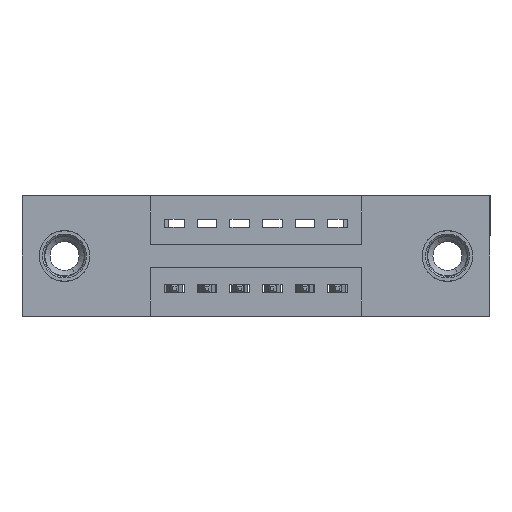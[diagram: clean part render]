
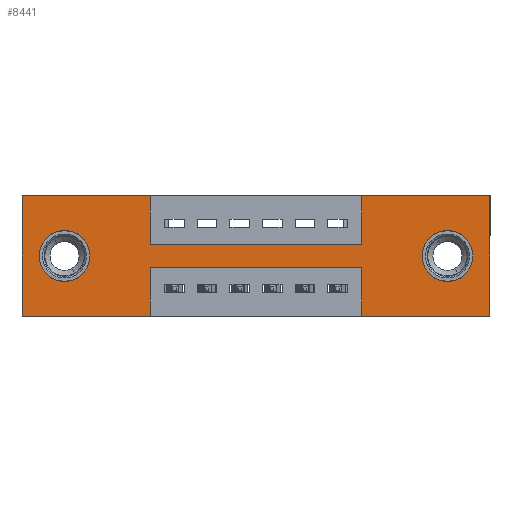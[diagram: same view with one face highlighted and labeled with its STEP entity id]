
A CAD part, front view. The second image highlights one B-rep face of the part: STEP entity #8441.
In plain terms, the highlighted planar face has unit normal (0, -1, 0).
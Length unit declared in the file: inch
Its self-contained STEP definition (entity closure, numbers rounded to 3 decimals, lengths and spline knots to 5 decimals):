
#17 = DIRECTION ( 'NONE',  ( 0., 0., 1. ) ) ;
#124 = DIRECTION ( 'NONE',  ( -1., 0., 0. ) ) ;
#183 = DIRECTION ( 'NONE',  ( -1., 0., 0. ) ) ;
#282 = EDGE_CURVE ( 'NONE', #2676, #2410, #8455, .T. ) ;
#309 = VERTEX_POINT ( 'NONE', #11609 ) ;
#420 = EDGE_CURVE ( 'NONE', #2410, #4218, #13909, .T. ) ;
#437 = EDGE_CURVE ( 'NONE', #10098, #4609, #4010, .T. ) ;
#442 = VERTEX_POINT ( 'NONE', #10493 ) ;
#476 = FACE_BOUND ( 'NONE', #6286, .T. ) ;
#587 = AXIS2_PLACEMENT_3D ( 'NONE', #9473, #10559, #1787 ) ;
#593 = LINE ( 'NONE', #3396, #13735 ) ;
#635 = FACE_OUTER_BOUND ( 'NONE', #5499, .T. ) ;
#681 = EDGE_CURVE ( 'NONE', #6985, #309, #10840, .T. ) ;
#711 = DIRECTION ( 'NONE',  ( 1., 0., 0. ) ) ;
#833 = FACE_BOUND ( 'NONE', #12904, .T. ) ;
#1046 = CARTESIAN_POINT ( 'NONE',  ( 1.0425, 0., 0. ) ) ;
#1182 = CARTESIAN_POINT ( 'NONE',  ( 0., 0., -0.37 ) ) ;
#1187 = DIRECTION ( 'NONE',  ( 0., 0., 1. ) ) ;
#1253 = EDGE_CURVE ( 'NONE', #4609, #10098, #2967, .T. ) ;
#1404 = CARTESIAN_POINT ( 'NONE',  ( 0.3925, 0., -0.15 ) ) ;
#1427 = EDGE_CURVE ( 'NONE', #4858, #3774, #3462, .T. ) ;
#1657 = VECTOR ( 'NONE', #2390, 39.37008 ) ;
#1787 = DIRECTION ( 'NONE',  ( 0., 0., -1. ) ) ;
#1828 = ORIENTED_EDGE ( 'NONE', *, *, #282, .F. ) ;
#1973 = VECTOR ( 'NONE', #4788, 39.37008 ) ;
#1985 = EDGE_CURVE ( 'NONE', #11065, #4858, #8744, .T. ) ;
#2332 = VECTOR ( 'NONE', #13837, 39.37008 ) ;
#2390 = DIRECTION ( 'NONE',  ( 1., 0., 0. ) ) ;
#2410 = VERTEX_POINT ( 'NONE', #1046 ) ;
#2585 = LINE ( 'NONE', #5685, #11122 ) ;
#2676 = VERTEX_POINT ( 'NONE', #9174 ) ;
#2867 = CARTESIAN_POINT ( 'NONE',  ( 0., 0., 0. ) ) ;
#2967 = CIRCLE ( 'NONE', #7599, 0.078 ) ;
#3246 = CARTESIAN_POINT ( 'NONE',  ( 0., 0., -0.37 ) ) ;
#3326 = VECTOR ( 'NONE', #711, 39.37008 ) ;
#3346 = ORIENTED_EDGE ( 'NONE', *, *, #12941, .F. ) ;
#3396 = CARTESIAN_POINT ( 'NONE',  ( 0.3925, 0., -0.37 ) ) ;
#3462 = LINE ( 'NONE', #5883, #8930 ) ;
#3595 = ORIENTED_EDGE ( 'NONE', *, *, #1253, .T. ) ;
#3707 = DIRECTION ( 'NONE',  ( 0., -1., 0. ) ) ;
#3774 = VERTEX_POINT ( 'NONE', #1404 ) ;
#4010 = CIRCLE ( 'NONE', #4722, 0.078 ) ;
#4049 = LINE ( 'NONE', #4590, #1657 ) ;
#4083 = CARTESIAN_POINT ( 'NONE',  ( 1.435, 0., 0. ) ) ;
#4100 = DIRECTION ( 'NONE',  ( 0., 0., -1. ) ) ;
#4122 = CARTESIAN_POINT ( 'NONE',  ( 0., 0., 0. ) ) ;
#4194 = CARTESIAN_POINT ( 'NONE',  ( 0.13, 0., -0.263 ) ) ;
#4218 = VERTEX_POINT ( 'NONE', #4695 ) ;
#4336 = VECTOR ( 'NONE', #11116, 39.37008 ) ;
#4443 = EDGE_CURVE ( 'NONE', #4218, #7850, #12376, .T. ) ;
#4590 = CARTESIAN_POINT ( 'NONE',  ( 0.3925, 0., -0.15 ) ) ;
#4609 = VERTEX_POINT ( 'NONE', #4194 ) ;
#4695 = CARTESIAN_POINT ( 'NONE',  ( 1.435, 0., 0. ) ) ;
#4713 = AXIS2_PLACEMENT_3D ( 'NONE', #8119, #3707, #11355 ) ;
#4722 = AXIS2_PLACEMENT_3D ( 'NONE', #9401, #10753, #17 ) ;
#4788 = DIRECTION ( 'NONE',  ( 0., 0., 1. ) ) ;
#4858 = VERTEX_POINT ( 'NONE', #8531 ) ;
#4966 = ORIENTED_EDGE ( 'NONE', *, *, #1427, .F. ) ;
#5242 = CARTESIAN_POINT ( 'NONE',  ( 1.305, 0., -0.185 ) ) ;
#5383 = DIRECTION ( 'NONE',  ( -1., 0., 0. ) ) ;
#5499 = EDGE_LOOP ( 'NONE', ( #9977, #6531, #3346, #6951, #11198, #11337, #1828, #7975, #4966, #8896, #6112, #6971 ) ) ;
#5592 = VECTOR ( 'NONE', #5383, 39.37008 ) ;
#5685 = CARTESIAN_POINT ( 'NONE',  ( 0., 0., -0.37 ) ) ;
#5883 = CARTESIAN_POINT ( 'NONE',  ( 0.3925, 0., 0. ) ) ;
#5970 = DIRECTION ( 'NONE',  ( 0., 0., -1. ) ) ;
#6006 = CIRCLE ( 'NONE', #10448, 0.078 ) ;
#6112 = ORIENTED_EDGE ( 'NONE', *, *, #11670, .F. ) ;
#6284 = VERTEX_POINT ( 'NONE', #3246 ) ;
#6286 = EDGE_LOOP ( 'NONE', ( #13090, #11822 ) ) ;
#6518 = CARTESIAN_POINT ( 'NONE',  ( 0., 0., 0. ) ) ;
#6529 = CARTESIAN_POINT ( 'NONE',  ( 0.3925, 0., -0.22 ) ) ;
#6531 = ORIENTED_EDGE ( 'NONE', *, *, #9839, .F. ) ;
#6649 = CARTESIAN_POINT ( 'NONE',  ( 1.0425, 0., -0.22 ) ) ;
#6775 = VECTOR ( 'NONE', #124, 39.37008 ) ;
#6841 = DIRECTION ( 'NONE',  ( 0., 0., 1. ) ) ;
#6951 = ORIENTED_EDGE ( 'NONE', *, *, #13366, .F. ) ;
#6971 = ORIENTED_EDGE ( 'NONE', *, *, #11247, .F. ) ;
#6985 = VERTEX_POINT ( 'NONE', #11508 ) ;
#7101 = EDGE_CURVE ( 'NONE', #309, #6985, #6006, .T. ) ;
#7599 = AXIS2_PLACEMENT_3D ( 'NONE', #11903, #13337, #6841 ) ;
#7850 = VERTEX_POINT ( 'NONE', #12219 ) ;
#7975 = ORIENTED_EDGE ( 'NONE', *, *, #10325, .F. ) ;
#8119 = CARTESIAN_POINT ( 'NONE',  ( 0., 0., -0.37 ) ) ;
#8441 = ADVANCED_FACE ( 'NONE', ( #476, #833, #635 ), #10254, .T. ) ;
#8455 = LINE ( 'NONE', #13683, #1973 ) ;
#8531 = CARTESIAN_POINT ( 'NONE',  ( 0.3925, 0., 0. ) ) ;
#8645 = LINE ( 'NONE', #6529, #5592 ) ;
#8647 = LINE ( 'NONE', #9000, #11374 ) ;
#8744 = LINE ( 'NONE', #6518, #4336 ) ;
#8896 = ORIENTED_EDGE ( 'NONE', *, *, #1985, .F. ) ;
#8930 = VECTOR ( 'NONE', #5970, 39.37008 ) ;
#9000 = CARTESIAN_POINT ( 'NONE',  ( 1.0425, 0., -0.37 ) ) ;
#9174 = CARTESIAN_POINT ( 'NONE',  ( 1.0425, 0., -0.15 ) ) ;
#9245 = VERTEX_POINT ( 'NONE', #9828 ) ;
#9299 = LINE ( 'NONE', #1182, #6775 ) ;
#9401 = CARTESIAN_POINT ( 'NONE',  ( 0.13, 0., -0.185 ) ) ;
#9473 = CARTESIAN_POINT ( 'NONE',  ( 1.305, 0., -0.185 ) ) ;
#9492 = CARTESIAN_POINT ( 'NONE',  ( 1.0425, 0., -0.37 ) ) ;
#9576 = CARTESIAN_POINT ( 'NONE',  ( 0., 0., 0. ) ) ;
#9680 = DIRECTION ( 'NONE',  ( 0., 1., 0. ) ) ;
#9828 = CARTESIAN_POINT ( 'NONE',  ( 0.3925, 0., -0.22 ) ) ;
#9839 = EDGE_CURVE ( 'NONE', #12851, #9245, #8645, .T. ) ;
#9947 = EDGE_CURVE ( 'NONE', #9245, #442, #593, .T. ) ;
#9977 = ORIENTED_EDGE ( 'NONE', *, *, #9947, .F. ) ;
#10098 = VERTEX_POINT ( 'NONE', #12351 ) ;
#10254 = PLANE ( 'NONE',  #4713 ) ;
#10325 = EDGE_CURVE ( 'NONE', #3774, #2676, #4049, .T. ) ;
#10381 = LINE ( 'NONE', #9576, #11416 ) ;
#10448 = AXIS2_PLACEMENT_3D ( 'NONE', #5242, #9680, #4100 ) ;
#10493 = CARTESIAN_POINT ( 'NONE',  ( 0.3925, 0., -0.37 ) ) ;
#10559 = DIRECTION ( 'NONE',  ( 0., 1., 0. ) ) ;
#10753 = DIRECTION ( 'NONE',  ( 0., 1., 0. ) ) ;
#10840 = CIRCLE ( 'NONE', #587, 0.078 ) ;
#11065 = VERTEX_POINT ( 'NONE', #4122 ) ;
#11116 = DIRECTION ( 'NONE',  ( 1., 0., 0. ) ) ;
#11122 = VECTOR ( 'NONE', #183, 39.37008 ) ;
#11198 = ORIENTED_EDGE ( 'NONE', *, *, #4443, .F. ) ;
#11247 = EDGE_CURVE ( 'NONE', #442, #6284, #2585, .T. ) ;
#11337 = ORIENTED_EDGE ( 'NONE', *, *, #420, .F. ) ;
#11355 = DIRECTION ( 'NONE',  ( 0., 0., -1. ) ) ;
#11374 = VECTOR ( 'NONE', #12203, 39.37008 ) ;
#11416 = VECTOR ( 'NONE', #1187, 39.37008 ) ;
#11508 = CARTESIAN_POINT ( 'NONE',  ( 1.305, 0., -0.107 ) ) ;
#11609 = CARTESIAN_POINT ( 'NONE',  ( 1.305, 0., -0.263 ) ) ;
#11670 = EDGE_CURVE ( 'NONE', #6284, #11065, #10381, .T. ) ;
#11822 = ORIENTED_EDGE ( 'NONE', *, *, #7101, .T. ) ;
#11903 = CARTESIAN_POINT ( 'NONE',  ( 0.13, 0., -0.185 ) ) ;
#12203 = DIRECTION ( 'NONE',  ( 0., 0., 1. ) ) ;
#12219 = CARTESIAN_POINT ( 'NONE',  ( 1.435, 0., -0.37 ) ) ;
#12351 = CARTESIAN_POINT ( 'NONE',  ( 0.13, 0., -0.107 ) ) ;
#12376 = LINE ( 'NONE', #4083, #2332 ) ;
#12619 = VERTEX_POINT ( 'NONE', #9492 ) ;
#12851 = VERTEX_POINT ( 'NONE', #6649 ) ;
#12866 = ORIENTED_EDGE ( 'NONE', *, *, #437, .T. ) ;
#12904 = EDGE_LOOP ( 'NONE', ( #12866, #3595 ) ) ;
#12941 = EDGE_CURVE ( 'NONE', #12619, #12851, #8647, .T. ) ;
#13090 = ORIENTED_EDGE ( 'NONE', *, *, #681, .T. ) ;
#13337 = DIRECTION ( 'NONE',  ( 0., 1., 0. ) ) ;
#13341 = DIRECTION ( 'NONE',  ( 0., 0., -1. ) ) ;
#13366 = EDGE_CURVE ( 'NONE', #7850, #12619, #9299, .T. ) ;
#13683 = CARTESIAN_POINT ( 'NONE',  ( 1.0425, 0., 0. ) ) ;
#13735 = VECTOR ( 'NONE', #13341, 39.37008 ) ;
#13837 = DIRECTION ( 'NONE',  ( 0., 0., -1. ) ) ;
#13909 = LINE ( 'NONE', #2867, #3326 ) ;
